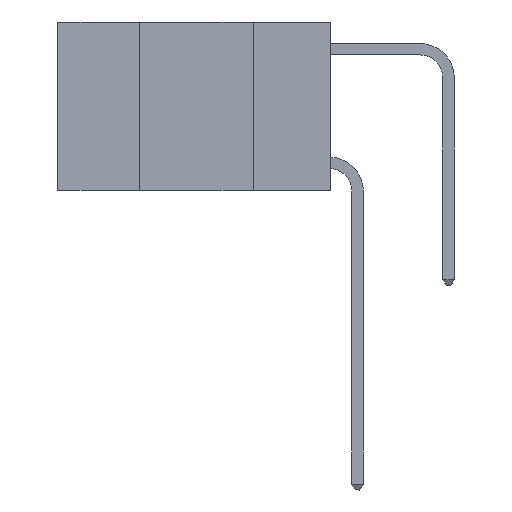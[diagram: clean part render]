
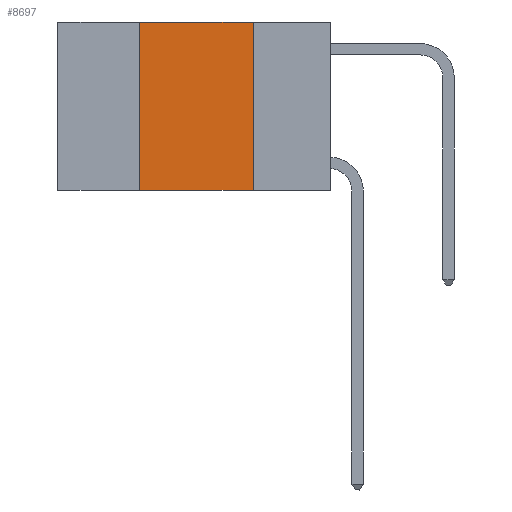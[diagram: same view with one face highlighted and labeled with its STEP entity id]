
A CAD part, left-side view. The second image highlights one B-rep face of the part: STEP entity #8697.
In plain terms, the highlighted planar face has unit normal (-1, 0, 0).
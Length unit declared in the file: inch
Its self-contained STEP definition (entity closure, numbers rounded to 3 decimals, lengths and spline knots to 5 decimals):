
#765 = EDGE_CURVE ( 'NONE', #26585, #10132, #17160, .T. ) ;
#802 = CARTESIAN_POINT ( 'NONE',  ( 0., 0.17, -0.37 ) ) ;
#814 = DIRECTION ( 'NONE',  ( 0., 0., 1. ) ) ;
#4415 = CARTESIAN_POINT ( 'NONE',  ( 0., 0.6, 0. ) ) ;
#4948 = EDGE_LOOP ( 'NONE', ( #9738, #9013, #5603, #11562 ) ) ;
#5603 = ORIENTED_EDGE ( 'NONE', *, *, #24012, .F. ) ;
#6519 = VECTOR ( 'NONE', #14923, 39.37008 ) ;
#6829 = DIRECTION ( 'NONE',  ( 0., 0., -1. ) ) ;
#8697 = ADVANCED_FACE ( 'NONE', ( #23939 ), #23368, .F. ) ;
#8816 = DIRECTION ( 'NONE',  ( 1., 0., 0. ) ) ;
#8843 = CARTESIAN_POINT ( 'NONE',  ( 0., 0.6, 0. ) ) ;
#9013 = ORIENTED_EDGE ( 'NONE', *, *, #10073, .F. ) ;
#9710 = CARTESIAN_POINT ( 'NONE',  ( 0., 0.42, 0. ) ) ;
#9738 = ORIENTED_EDGE ( 'NONE', *, *, #765, .F. ) ;
#10073 = EDGE_CURVE ( 'NONE', #19497, #26585, #25852, .T. ) ;
#10132 = VERTEX_POINT ( 'NONE', #802 ) ;
#11562 = ORIENTED_EDGE ( 'NONE', *, *, #16433, .T. ) ;
#13221 = VECTOR ( 'NONE', #25112, 39.37008 ) ;
#13367 = DIRECTION ( 'NONE',  ( 0., -1., 0. ) ) ;
#14817 = VECTOR ( 'NONE', #814, 39.37008 ) ;
#14923 = DIRECTION ( 'NONE',  ( 0., -1., 0. ) ) ;
#15406 = CARTESIAN_POINT ( 'NONE',  ( 0., 0.17, 0. ) ) ;
#15457 = LINE ( 'NONE', #26053, #14817 ) ;
#16273 = CARTESIAN_POINT ( 'NONE',  ( 0., 0.42, -0.37 ) ) ;
#16433 = EDGE_CURVE ( 'NONE', #25408, #10132, #19404, .T. ) ;
#16971 = VECTOR ( 'NONE', #13367, 39.37008 ) ;
#17160 = LINE ( 'NONE', #20696, #13221 ) ;
#18789 = CARTESIAN_POINT ( 'NONE',  ( 0., 0.6, -0.37 ) ) ;
#19404 = LINE ( 'NONE', #18789, #6519 ) ;
#19497 = VERTEX_POINT ( 'NONE', #9710 ) ;
#20696 = CARTESIAN_POINT ( 'NONE',  ( 0., 0.17, 0. ) ) ;
#22438 = AXIS2_PLACEMENT_3D ( 'NONE', #4415, #8816, #6829 ) ;
#23368 = PLANE ( 'NONE',  #22438 ) ;
#23939 = FACE_OUTER_BOUND ( 'NONE', #4948, .T. ) ;
#24012 = EDGE_CURVE ( 'NONE', #25408, #19497, #15457, .T. ) ;
#25112 = DIRECTION ( 'NONE',  ( 0., 0., -1. ) ) ;
#25408 = VERTEX_POINT ( 'NONE', #16273 ) ;
#25852 = LINE ( 'NONE', #8843, #16971 ) ;
#26053 = CARTESIAN_POINT ( 'NONE',  ( 0., 0.42, 0. ) ) ;
#26585 = VERTEX_POINT ( 'NONE', #15406 ) ;
